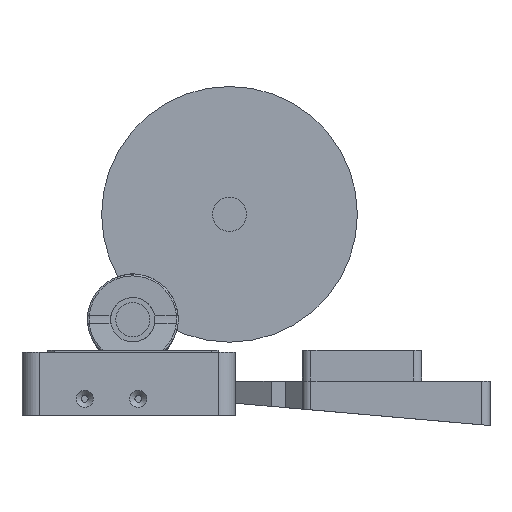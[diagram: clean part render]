
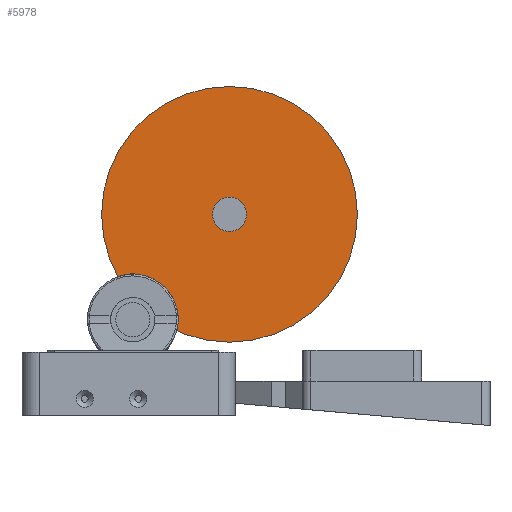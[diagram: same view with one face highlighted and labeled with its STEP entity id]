
A CAD part, front view. The second image highlights one B-rep face of the part: STEP entity #5978.
In plain terms, the highlighted planar face has unit normal (0, -1, 0).
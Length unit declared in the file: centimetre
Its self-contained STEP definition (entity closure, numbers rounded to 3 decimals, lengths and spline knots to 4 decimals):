
#1289=PLANE($,#6379);
#1593=FACE_BOUND($,#2136,.T.);
#1594=FACE_BOUND($,#2137,.T.);
#2136=EDGE_LOOP($,(#4500));
#2137=EDGE_LOOP($,(#4501));
#2520=CIRCLE($,#6373,1.);
#2521=CIRCLE($,#6377,7.5);
#2786=VERTEX_POINT($,#10239);
#2787=VERTEX_POINT($,#10244);
#3441=EDGE_CURVE($,#2786,#2786,#2520,.T.);
#3442=EDGE_CURVE($,#2787,#2787,#2521,.T.);
#4500=ORIENTED_EDGE($,*,*,#3441,.T.);
#4501=ORIENTED_EDGE($,*,*,#3442,.T.);
#5978=ADVANCED_FACE($,(#1593,#1594),#1289,.T.);
#6373=AXIS2_PLACEMENT_3D($,#10240,#7094,#7095);
#6377=AXIS2_PLACEMENT_3D($,#10245,#7102,#7103);
#6379=AXIS2_PLACEMENT_3D($,#10248,#7106,#7107);
#7094=DIRECTION('center_axis',(0.,1.,0.));
#7095=DIRECTION('ref_axis',(1.,0.,0.));
#7102=DIRECTION('center_axis',(0.,-1.,0.));
#7103=DIRECTION('ref_axis',(1.,0.,0.));
#7106=DIRECTION('center_axis',(0.,-1.,0.));
#7107=DIRECTION('ref_axis',(-1.,0.,0.));
#10239=CARTESIAN_POINT('',(4.6714,7.325,10.7793));
#10240=CARTESIAN_POINT('Origin',(5.6714,7.325,10.7793));
#10244=CARTESIAN_POINT('',(13.1714,7.325,10.7793));
#10245=CARTESIAN_POINT('Origin',(5.6714,7.325,10.7793));
#10248=CARTESIAN_POINT('Origin',(5.6714,7.325,10.7793));
